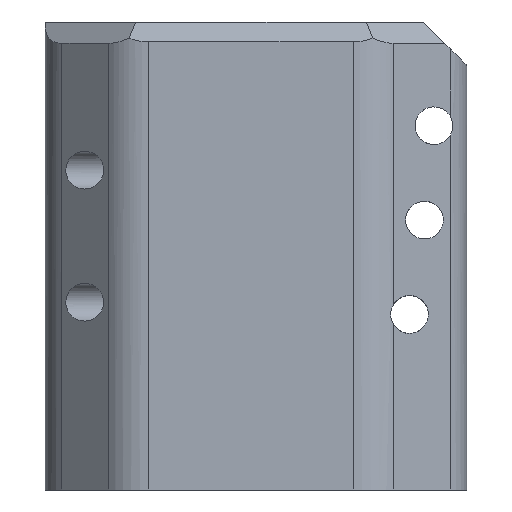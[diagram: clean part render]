
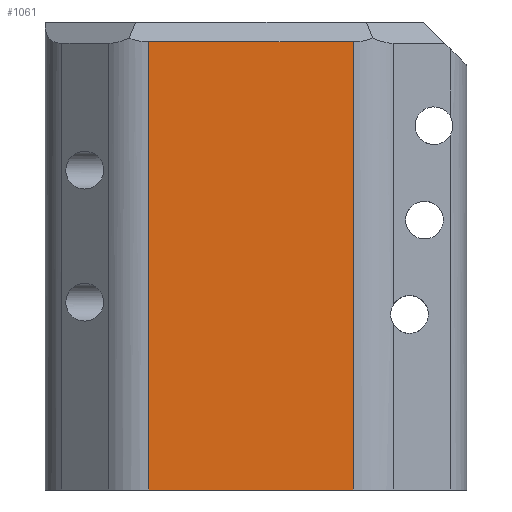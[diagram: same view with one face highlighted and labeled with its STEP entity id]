
A CAD part, left-side view. The second image highlights one B-rep face of the part: STEP entity #1061.
In plain terms, the highlighted planar face has unit normal (-1, 0, 0).
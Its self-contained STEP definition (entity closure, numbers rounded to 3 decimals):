
#51=LINE('',#2175,#102);
#69=LINE('',#2436,#120);
#86=LINE('',#2515,#137);
#87=LINE('',#2517,#138);
#102=VECTOR('',#1337,10.);
#120=VECTOR('',#1443,10.);
#137=VECTOR('',#1496,10.);
#138=VECTOR('',#1499,10.);
#173=PLANE('',#1205);
#241=FACE_OUTER_BOUND('',#304,.T.);
#304=EDGE_LOOP('',(#965,#966,#967,#968));
#462=VERTEX_POINT('',#2172);
#463=VERTEX_POINT('',#2174);
#495=VERTEX_POINT('',#2433);
#496=VERTEX_POINT('',#2435);
#590=EDGE_CURVE('',#463,#462,#51,.F.);
#642=EDGE_CURVE('',#496,#495,#69,.F.);
#670=EDGE_CURVE('',#462,#496,#86,.T.);
#671=EDGE_CURVE('',#495,#463,#87,.T.);
#965=ORIENTED_EDGE('',*,*,#671,.T.);
#966=ORIENTED_EDGE('',*,*,#590,.T.);
#967=ORIENTED_EDGE('',*,*,#670,.T.);
#968=ORIENTED_EDGE('',*,*,#642,.T.);
#1061=ADVANCED_FACE('',(#241),#173,.F.);
#1205=AXIS2_PLACEMENT_3D('',#2516,#1497,#1498);
#1337=DIRECTION('',(0.,1.,0.));
#1443=DIRECTION('',(0.,-1.,0.));
#1496=DIRECTION('',(0.,0.,1.));
#1497=DIRECTION('center_axis',(1.,0.,0.));
#1498=DIRECTION('ref_axis',(0.,1.,0.));
#1499=DIRECTION('',(0.,0.,-1.));
#2172=CARTESIAN_POINT('',(-26.04,-37.501,-61.002));
#2174=CARTESIAN_POINT('',(-26.04,-15.843,-61.002));
#2175=CARTESIAN_POINT('',(-26.04,-22.962,-61.002));
#2433=CARTESIAN_POINT('',(-26.04,-15.843,-13.514));
#2435=CARTESIAN_POINT('',(-26.04,-37.501,-13.514));
#2436=CARTESIAN_POINT('',(-26.04,-30.676,-13.514));
#2515=CARTESIAN_POINT('',(-26.04,-37.501,-45.707));
#2516=CARTESIAN_POINT('Origin',(-26.04,-40.043,-54.648));
#2517=CARTESIAN_POINT('',(-26.04,-15.843,-54.648));
